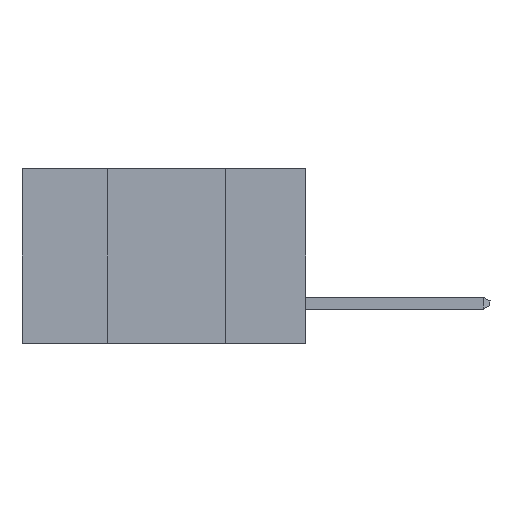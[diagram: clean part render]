
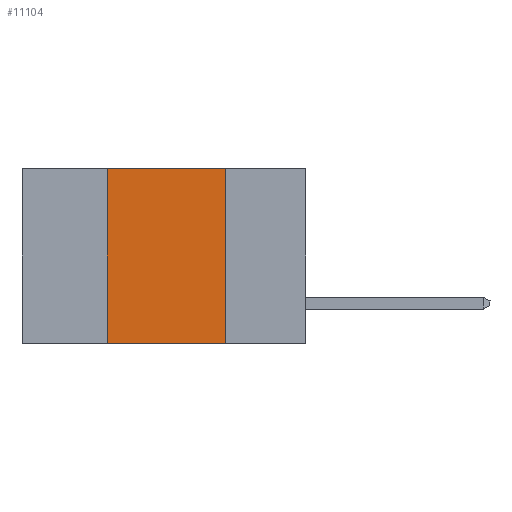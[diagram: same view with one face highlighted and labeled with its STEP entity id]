
A CAD part, left-side view. The second image highlights one B-rep face of the part: STEP entity #11104.
In plain terms, the highlighted planar face has unit normal (-1, 0, 0).
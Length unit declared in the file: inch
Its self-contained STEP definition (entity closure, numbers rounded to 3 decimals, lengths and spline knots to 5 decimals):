
#808 = FACE_OUTER_BOUND ( 'NONE', #1021, .T. ) ;
#1021 = EDGE_LOOP ( 'NONE', ( #10254, #8685, #6588, #2375 ) ) ;
#1149 = LINE ( 'NONE', #12203, #1400 ) ;
#1400 = VECTOR ( 'NONE', #9886, 39.37008 ) ;
#1962 = PLANE ( 'NONE',  #5513 ) ;
#2049 = VERTEX_POINT ( 'NONE', #10508 ) ;
#2375 = ORIENTED_EDGE ( 'NONE', *, *, #3759, .T. ) ;
#2585 = VECTOR ( 'NONE', #13084, 39.37008 ) ;
#2962 = LINE ( 'NONE', #6377, #7355 ) ;
#3759 = EDGE_CURVE ( 'NONE', #3900, #2049, #4484, .T. ) ;
#3843 = CARTESIAN_POINT ( 'NONE',  ( 0., 0.42, 0. ) ) ;
#3900 = VERTEX_POINT ( 'NONE', #11351 ) ;
#4123 = DIRECTION ( 'NONE',  ( 1., 0., 0. ) ) ;
#4484 = LINE ( 'NONE', #7733, #2585 ) ;
#4779 = CARTESIAN_POINT ( 'NONE',  ( 0., 0.6, 0. ) ) ;
#5214 = CARTESIAN_POINT ( 'NONE',  ( 0., 0.6, 0. ) ) ;
#5513 = AXIS2_PLACEMENT_3D ( 'NONE', #5214, #4123, #12941 ) ;
#6377 = CARTESIAN_POINT ( 'NONE',  ( 0., 0.42, -0.37 ) ) ;
#6588 = ORIENTED_EDGE ( 'NONE', *, *, #10594, .F. ) ;
#7179 = CARTESIAN_POINT ( 'NONE',  ( 0., 0.17, 0. ) ) ;
#7331 = VERTEX_POINT ( 'NONE', #3843 ) ;
#7355 = VECTOR ( 'NONE', #11933, 39.37008 ) ;
#7733 = CARTESIAN_POINT ( 'NONE',  ( 0., 0.6, -0.37 ) ) ;
#8685 = ORIENTED_EDGE ( 'NONE', *, *, #10567, .F. ) ;
#9029 = VECTOR ( 'NONE', #12517, 39.37008 ) ;
#9886 = DIRECTION ( 'NONE',  ( 0., 0., -1. ) ) ;
#10254 = ORIENTED_EDGE ( 'NONE', *, *, #12959, .F. ) ;
#10508 = CARTESIAN_POINT ( 'NONE',  ( 0., 0.17, -0.37 ) ) ;
#10567 = EDGE_CURVE ( 'NONE', #7331, #12799, #12802, .T. ) ;
#10594 = EDGE_CURVE ( 'NONE', #3900, #7331, #2962, .T. ) ;
#11104 = ADVANCED_FACE ( 'NONE', ( #808 ), #1962, .F. ) ;
#11351 = CARTESIAN_POINT ( 'NONE',  ( 0., 0.42, -0.37 ) ) ;
#11933 = DIRECTION ( 'NONE',  ( 0., 0., 1. ) ) ;
#12203 = CARTESIAN_POINT ( 'NONE',  ( 0., 0.17, -0.37 ) ) ;
#12517 = DIRECTION ( 'NONE',  ( 0., -1., 0. ) ) ;
#12799 = VERTEX_POINT ( 'NONE', #7179 ) ;
#12802 = LINE ( 'NONE', #4779, #9029 ) ;
#12941 = DIRECTION ( 'NONE',  ( 0., 0., -1. ) ) ;
#12959 = EDGE_CURVE ( 'NONE', #12799, #2049, #1149, .T. ) ;
#13084 = DIRECTION ( 'NONE',  ( 0., -1., 0. ) ) ;
